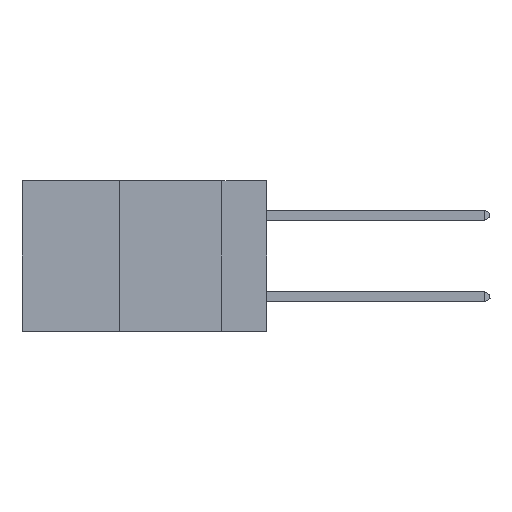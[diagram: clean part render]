
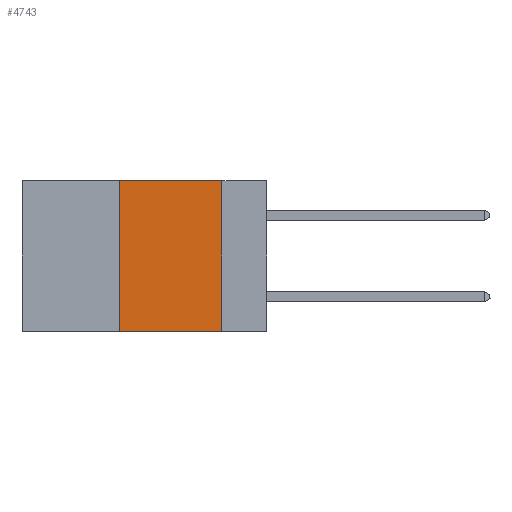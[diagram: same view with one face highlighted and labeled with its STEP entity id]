
A CAD part, left-side view. The second image highlights one B-rep face of the part: STEP entity #4743.
In plain terms, the highlighted planar face has unit normal (-1, 0, 0).
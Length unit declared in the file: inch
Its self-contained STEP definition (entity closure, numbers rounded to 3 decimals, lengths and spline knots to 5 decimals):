
#173 = VERTEX_POINT ( 'NONE', #4783 ) ;
#280 = ORIENTED_EDGE ( 'NONE', *, *, #14003, .F. ) ;
#298 = EDGE_CURVE ( 'NONE', #173, #15244, #6015, .T. ) ;
#873 = CARTESIAN_POINT ( 'NONE',  ( 0., 0.36, 0. ) ) ;
#2405 = DIRECTION ( 'NONE',  ( 0., 0., 1. ) ) ;
#2413 = VECTOR ( 'NONE', #2405, 39.37008 ) ;
#2813 = LINE ( 'NONE', #16419, #17050 ) ;
#3605 = DIRECTION ( 'NONE',  ( 1., 0., 0. ) ) ;
#4743 = ADVANCED_FACE ( 'NONE', ( #7407 ), #11984, .F. ) ;
#4783 = CARTESIAN_POINT ( 'NONE',  ( 0., 0.36, -0.37 ) ) ;
#4917 = VERTEX_POINT ( 'NONE', #13633 ) ;
#5508 = LINE ( 'NONE', #15423, #16012 ) ;
#5526 = DIRECTION ( 'NONE',  ( 0., 0., -1. ) ) ;
#5702 = DIRECTION ( 'NONE',  ( 0., -1., 0. ) ) ;
#5929 = ORIENTED_EDGE ( 'NONE', *, *, #8562, .F. ) ;
#6015 = LINE ( 'NONE', #10042, #16910 ) ;
#6237 = LINE ( 'NONE', #873, #2413 ) ;
#7115 = VERTEX_POINT ( 'NONE', #12966 ) ;
#7407 = FACE_OUTER_BOUND ( 'NONE', #8774, .T. ) ;
#7436 = ORIENTED_EDGE ( 'NONE', *, *, #12456, .F. ) ;
#7820 = CARTESIAN_POINT ( 'NONE',  ( 0., 0.11, -0.37 ) ) ;
#7831 = CARTESIAN_POINT ( 'NONE',  ( 0., 0.6, 0. ) ) ;
#8562 = EDGE_CURVE ( 'NONE', #4917, #15244, #2813, .T. ) ;
#8774 = EDGE_LOOP ( 'NONE', ( #5929, #280, #7436, #15731 ) ) ;
#10042 = CARTESIAN_POINT ( 'NONE',  ( 0., 0.6, -0.37 ) ) ;
#11984 = PLANE ( 'NONE',  #12001 ) ;
#12001 = AXIS2_PLACEMENT_3D ( 'NONE', #7831, #3605, #13323 ) ;
#12456 = EDGE_CURVE ( 'NONE', #173, #7115, #6237, .T. ) ;
#12966 = CARTESIAN_POINT ( 'NONE',  ( 0., 0.36, 0. ) ) ;
#13323 = DIRECTION ( 'NONE',  ( 0., 0., -1. ) ) ;
#13633 = CARTESIAN_POINT ( 'NONE',  ( 0., 0.11, 0. ) ) ;
#14003 = EDGE_CURVE ( 'NONE', #7115, #4917, #5508, .T. ) ;
#15244 = VERTEX_POINT ( 'NONE', #7820 ) ;
#15423 = CARTESIAN_POINT ( 'NONE',  ( 0., 0.6, 0. ) ) ;
#15731 = ORIENTED_EDGE ( 'NONE', *, *, #298, .T. ) ;
#16012 = VECTOR ( 'NONE', #16758, 39.37008 ) ;
#16419 = CARTESIAN_POINT ( 'NONE',  ( 0., 0.11, 0. ) ) ;
#16758 = DIRECTION ( 'NONE',  ( 0., -1., 0. ) ) ;
#16910 = VECTOR ( 'NONE', #5702, 39.37008 ) ;
#17050 = VECTOR ( 'NONE', #5526, 39.37008 ) ;
